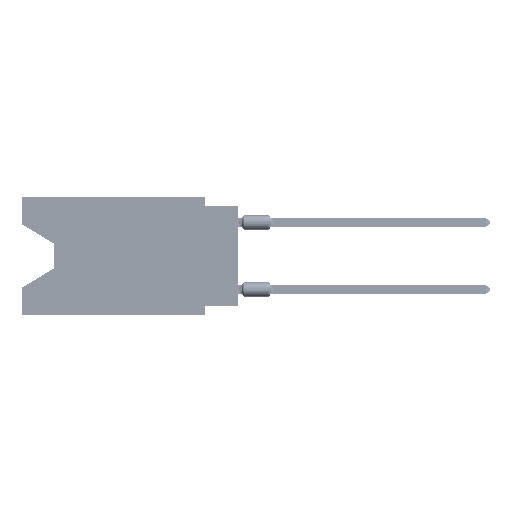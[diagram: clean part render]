
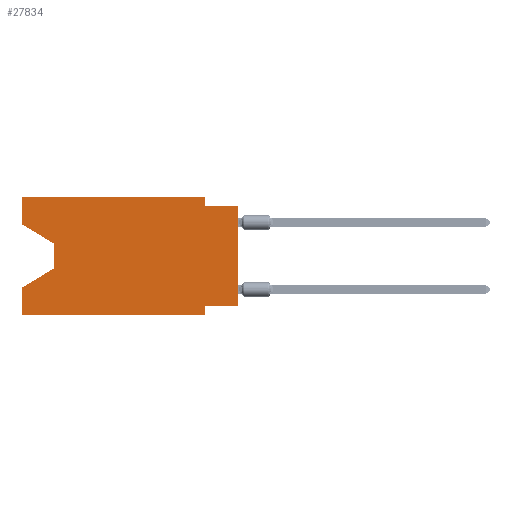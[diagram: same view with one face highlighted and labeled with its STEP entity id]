
A CAD part, left-side view. The second image highlights one B-rep face of the part: STEP entity #27834.
In plain terms, the highlighted planar face has unit normal (-1, 0, 0).
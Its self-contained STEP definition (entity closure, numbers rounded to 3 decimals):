
#1227 = DIRECTION ( 'NONE',  ( 0., 0., -1. ) ) ;
#1260 = DIRECTION ( 'NONE',  ( 0., 0., -1. ) ) ;
#1444 = VERTEX_POINT ( 'NONE', #26926 ) ;
#1599 = DIRECTION ( 'NONE',  ( 0., -0.855, -0.519 ) ) ;
#1923 = CARTESIAN_POINT ( 'NONE',  ( 0., 0., -0.635 ) ) ;
#1991 = ORIENTED_EDGE ( 'NONE', *, *, #81978, .F. ) ;
#2027 = CARTESIAN_POINT ( 'NONE',  ( 0., 2.54, 0. ) ) ;
#2391 = DIRECTION ( 'NONE',  ( 0., 0., 1. ) ) ;
#3936 = CARTESIAN_POINT ( 'NONE',  ( 0., 0., -8.255 ) ) ;
#5638 = CARTESIAN_POINT ( 'NONE',  ( 0., 2.54, -8.255 ) ) ;
#6874 = DIRECTION ( 'NONE',  ( 1., 0., 0. ) ) ;
#6949 = CARTESIAN_POINT ( 'NONE',  ( 0., 16.383, 0. ) ) ;
#8275 = CARTESIAN_POINT ( 'NONE',  ( 0., 16.383, 0. ) ) ;
#9599 = AXIS2_PLACEMENT_3D ( 'NONE', #8275, #6874, #57246 ) ;
#9605 = VECTOR ( 'NONE', #17723, 1000. ) ;
#11272 = EDGE_CURVE ( 'NONE', #17261, #70466, #22176, .T. ) ;
#11878 = EDGE_CURVE ( 'NONE', #26779, #28591, #38196, .T. ) ;
#11991 = DIRECTION ( 'NONE',  ( 0., 0.855, -0.519 ) ) ;
#12914 = ORIENTED_EDGE ( 'NONE', *, *, #89738, .T. ) ;
#17232 = LINE ( 'NONE', #3936, #64829 ) ;
#17261 = VERTEX_POINT ( 'NONE', #5638 ) ;
#17723 = DIRECTION ( 'NONE',  ( 0., 0., -1. ) ) ;
#17767 = VECTOR ( 'NONE', #1260, 1000. ) ;
#21508 = CARTESIAN_POINT ( 'NONE',  ( 0., 13.97, -5.385 ) ) ;
#22176 = LINE ( 'NONE', #35980, #17767 ) ;
#22437 = VECTOR ( 'NONE', #68448, 1000. ) ;
#22775 = ORIENTED_EDGE ( 'NONE', *, *, #28028, .F. ) ;
#23208 = DIRECTION ( 'NONE',  ( 0., -1., 0. ) ) ;
#24713 = CARTESIAN_POINT ( 'NONE',  ( 0., 0., 0. ) ) ;
#25773 = EDGE_CURVE ( 'NONE', #71435, #70466, #82918, .T. ) ;
#26607 = ORIENTED_EDGE ( 'NONE', *, *, #55756, .F. ) ;
#26779 = VERTEX_POINT ( 'NONE', #89917 ) ;
#26821 = EDGE_CURVE ( 'NONE', #65484, #68173, #74744, .T. ) ;
#26926 = CARTESIAN_POINT ( 'NONE',  ( 0., 0., -8.255 ) ) ;
#27834 = ADVANCED_FACE ( 'NONE', ( #59115 ), #43447, .F. ) ;
#28028 = EDGE_CURVE ( 'NONE', #48067, #65484, #31524, .T. ) ;
#28591 = VERTEX_POINT ( 'NONE', #47551 ) ;
#30897 = LINE ( 'NONE', #81742, #76185 ) ;
#31524 = LINE ( 'NONE', #45323, #33901 ) ;
#33901 = VECTOR ( 'NONE', #74310, 1000. ) ;
#34229 = VERTEX_POINT ( 'NONE', #21508 ) ;
#35546 = ORIENTED_EDGE ( 'NONE', *, *, #11878, .T. ) ;
#35980 = CARTESIAN_POINT ( 'NONE',  ( 0., 2.54, -8.89 ) ) ;
#36048 = ORIENTED_EDGE ( 'NONE', *, *, #44298, .F. ) ;
#37008 = LINE ( 'NONE', #87842, #56962 ) ;
#38196 = LINE ( 'NONE', #60066, #78548 ) ;
#38751 = CARTESIAN_POINT ( 'NONE',  ( 0., 16.383, -8.89 ) ) ;
#40050 = DIRECTION ( 'NONE',  ( 0., 1., 0. ) ) ;
#42333 = EDGE_LOOP ( 'NONE', ( #35546, #87273, #12914, #70588, #56671, #91345, #36048, #61698, #1991, #77642, #22775, #26607 ) ) ;
#43447 = PLANE ( 'NONE',  #9599 ) ;
#43744 = EDGE_CURVE ( 'NONE', #28591, #34229, #79634, .T. ) ;
#44298 = EDGE_CURVE ( 'NONE', #1444, #17261, #17232, .T. ) ;
#44384 = CARTESIAN_POINT ( 'NONE',  ( 0., 16.383, -8.89 ) ) ;
#44773 = EDGE_CURVE ( 'NONE', #1444, #81564, #88403, .T. ) ;
#45323 = CARTESIAN_POINT ( 'NONE',  ( 0., 16.383, 0. ) ) ;
#45410 = CARTESIAN_POINT ( 'NONE',  ( 0., 13.97, -3.505 ) ) ;
#45855 = DIRECTION ( 'NONE',  ( 0., -1., 0. ) ) ;
#45956 = CARTESIAN_POINT ( 'NONE',  ( 0., 16.383, 0. ) ) ;
#47551 = CARTESIAN_POINT ( 'NONE',  ( 0., 13.97, -3.505 ) ) ;
#48067 = VERTEX_POINT ( 'NONE', #6949 ) ;
#48452 = EDGE_CURVE ( 'NONE', #71435, #82080, #30897, .T. ) ;
#52635 = VECTOR ( 'NONE', #11991, 1000. ) ;
#53515 = CARTESIAN_POINT ( 'NONE',  ( 0., 2.54, -0.635 ) ) ;
#55756 = EDGE_CURVE ( 'NONE', #26779, #48067, #62108, .T. ) ;
#56671 = ORIENTED_EDGE ( 'NONE', *, *, #25773, .T. ) ;
#56962 = VECTOR ( 'NONE', #23208, 1000. ) ;
#57246 = DIRECTION ( 'NONE',  ( 0., 0., -1. ) ) ;
#57898 = LINE ( 'NONE', #86851, #52635 ) ;
#59115 = FACE_OUTER_BOUND ( 'NONE', #42333, .T. ) ;
#60066 = CARTESIAN_POINT ( 'NONE',  ( 0., 16.383, -2.038 ) ) ;
#61216 = CARTESIAN_POINT ( 'NONE',  ( 0., 16.383, -6.852 ) ) ;
#61698 = ORIENTED_EDGE ( 'NONE', *, *, #44773, .T. ) ;
#62108 = LINE ( 'NONE', #45956, #73497 ) ;
#64829 = VECTOR ( 'NONE', #40050, 1000. ) ;
#65484 = VERTEX_POINT ( 'NONE', #92022 ) ;
#68173 = VERTEX_POINT ( 'NONE', #53515 ) ;
#68448 = DIRECTION ( 'NONE',  ( 0., 0., 1. ) ) ;
#70466 = VERTEX_POINT ( 'NONE', #86451 ) ;
#70588 = ORIENTED_EDGE ( 'NONE', *, *, #48452, .F. ) ;
#71435 = VERTEX_POINT ( 'NONE', #44384 ) ;
#73497 = VECTOR ( 'NONE', #91081, 1000. ) ;
#74310 = DIRECTION ( 'NONE',  ( 0., -1., 0. ) ) ;
#74744 = LINE ( 'NONE', #2027, #9605 ) ;
#76185 = VECTOR ( 'NONE', #2391, 1000. ) ;
#77642 = ORIENTED_EDGE ( 'NONE', *, *, #26821, .F. ) ;
#78548 = VECTOR ( 'NONE', #1599, 1000. ) ;
#79634 = LINE ( 'NONE', #45410, #93592 ) ;
#80817 = VECTOR ( 'NONE', #45855, 1000. ) ;
#81564 = VERTEX_POINT ( 'NONE', #1923 ) ;
#81742 = CARTESIAN_POINT ( 'NONE',  ( 0., 16.383, 0. ) ) ;
#81978 = EDGE_CURVE ( 'NONE', #68173, #81564, #37008, .T. ) ;
#82080 = VERTEX_POINT ( 'NONE', #61216 ) ;
#82918 = LINE ( 'NONE', #38751, #80817 ) ;
#86451 = CARTESIAN_POINT ( 'NONE',  ( 0., 2.54, -8.89 ) ) ;
#86851 = CARTESIAN_POINT ( 'NONE',  ( 0., 13.97, -5.385 ) ) ;
#87273 = ORIENTED_EDGE ( 'NONE', *, *, #43744, .T. ) ;
#87842 = CARTESIAN_POINT ( 'NONE',  ( 0., 0., -0.635 ) ) ;
#88403 = LINE ( 'NONE', #24713, #22437 ) ;
#89738 = EDGE_CURVE ( 'NONE', #34229, #82080, #57898, .T. ) ;
#89917 = CARTESIAN_POINT ( 'NONE',  ( 0., 16.383, -2.038 ) ) ;
#91081 = DIRECTION ( 'NONE',  ( 0., 0., 1. ) ) ;
#91345 = ORIENTED_EDGE ( 'NONE', *, *, #11272, .F. ) ;
#92022 = CARTESIAN_POINT ( 'NONE',  ( 0., 2.54, 0. ) ) ;
#93592 = VECTOR ( 'NONE', #1227, 1000. ) ;
